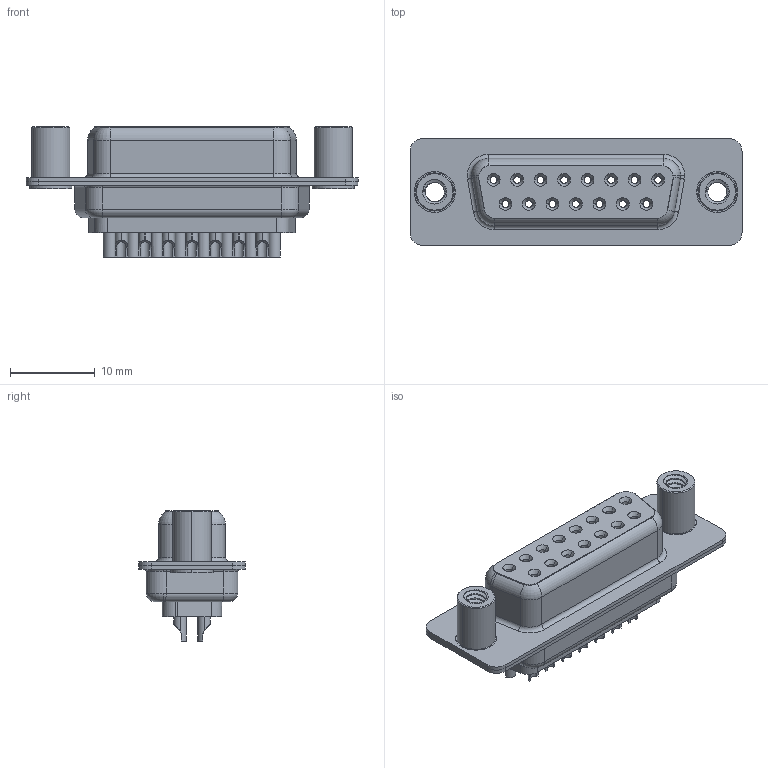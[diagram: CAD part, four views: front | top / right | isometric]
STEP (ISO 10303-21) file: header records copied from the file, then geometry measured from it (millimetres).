
FILE_DESCRIPTION (( 'STEP AP203' ), '1' );
FILE_NAME ('628-015-622-268.STEP', '2020-07-14T03:43:51', ( '' ), ( '' ), 'SwSTEP 2.0', 'SolidWorks 2020', '' );
FILE_SCHEMA (( 'CONFIG_CONTROL_DESIGN' ));
Length unit declared in the file: millimetre
Products named in the file (7): 628-015-622-268; 628 Housing_15 LP; 628 Shell Front_15 Contacts; 628 Contact Row 2_22L; 628 Contact Row 1_22L; 628 Shell Rear_15 Contacts; 628 4-40 Threaded Standoff
Assembly tree (20 placements, depth 2):
  628-015-622-268
    628 Housing_15 LP
    628 Shell Front_15 Contacts
    628 Shell Rear_15 Contacts
    628 Contact Row 1_22L  x8
    628 Contact Row 2_22L  x7
    628 4-40 Threaded Standoff  x2
Bounding box: 39.15 x 12.6 x 15.35 mm (x, y, z)
Volume: 2611.9 mm3; surface area: 6553.3 mm2
Topology: 20 solids, 20 shells, 1648 faces, 4169 edges, 2619 vertices
Faces by surface type: cylinder 540, plane 384, torus 333, bspline 306, cone 85
Entity records: 22246 total; most frequent: CARTESIAN_POINT 6910, DIRECTION 3079, ORIENTED_EDGE 2934, EDGE_CURVE 1467, AXIS2_PLACEMENT_3D 1279, VERTEX_POINT 924, EDGE_LOOP 709, CIRCLE 689
